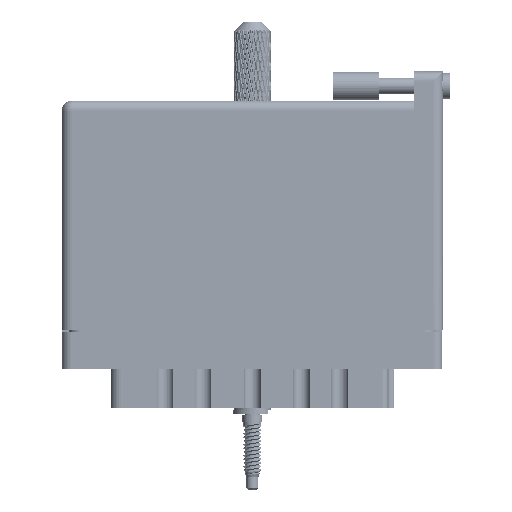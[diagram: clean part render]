
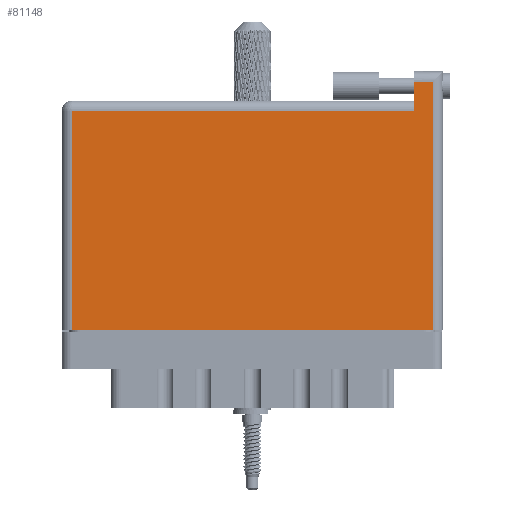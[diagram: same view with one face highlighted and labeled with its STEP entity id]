
A CAD part, front view. The second image highlights one B-rep face of the part: STEP entity #81148.
In plain terms, the highlighted face is planar.
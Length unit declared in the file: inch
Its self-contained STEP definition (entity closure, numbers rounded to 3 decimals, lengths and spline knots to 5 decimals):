
#1826 = AXIS2_PLACEMENT_3D ( 'NONE', #82770, #83542, #58306 ) ;
#6458 = ORIENTED_EDGE ( 'NONE', *, *, #20138, .T. ) ;
#6482 = CARTESIAN_POINT ( 'NONE',  ( 2.53, 1.696, 0. ) ) ;
#8114 = VERTEX_POINT ( 'NONE', #28756 ) ;
#8394 = VERTEX_POINT ( 'NONE', #106217 ) ;
#8810 = EDGE_LOOP ( 'NONE', ( #108241, #108250, #6458, #107707, #86472, #81089 ) ) ;
#10524 = VERTEX_POINT ( 'NONE', #55354 ) ;
#12526 = DIRECTION ( 'NONE',  ( 0., 1., 0. ) ) ;
#14094 = CARTESIAN_POINT ( 'NONE',  ( 0.07, 0., 0. ) ) ;
#14595 = LINE ( 'NONE', #22500, #80674 ) ;
#17447 = DIRECTION ( 'NONE',  ( 0., -1., 0. ) ) ;
#20138 = EDGE_CURVE ( 'NONE', #86736, #8394, #29441, .T. ) ;
#22500 = CARTESIAN_POINT ( 'NONE',  ( 2.53, 1.766, 0. ) ) ;
#27860 = LINE ( 'NONE', #66190, #40802 ) ;
#28756 = CARTESIAN_POINT ( 'NONE',  ( 2.53, 0., 0. ) ) ;
#29441 = LINE ( 'NONE', #54381, #75529 ) ;
#33215 = VERTEX_POINT ( 'NONE', #49548 ) ;
#36217 = LINE ( 'NONE', #70089, #112387 ) ;
#38196 = LINE ( 'NONE', #14094, #77032 ) ;
#40200 = DIRECTION ( 'NONE',  ( 0., -1., 0. ) ) ;
#40802 = VECTOR ( 'NONE', #86658, 39.37008 ) ;
#43495 = EDGE_CURVE ( 'NONE', #10524, #49974, #38196, .T. ) ;
#49107 = PLANE ( 'NONE',  #1826 ) ;
#49548 = CARTESIAN_POINT ( 'NONE',  ( 2.403, 1.496, 0. ) ) ;
#49974 = VERTEX_POINT ( 'NONE', #74102 ) ;
#53403 = VECTOR ( 'NONE', #75954, 39.37008 ) ;
#54381 = CARTESIAN_POINT ( 'NONE',  ( 0., 1.696, 0. ) ) ;
#54705 = FACE_OUTER_BOUND ( 'NONE', #8810, .T. ) ;
#55354 = CARTESIAN_POINT ( 'NONE',  ( 0.07, 1.496, 0. ) ) ;
#57120 = CARTESIAN_POINT ( 'NONE',  ( 0., 1.496, 0. ) ) ;
#58306 = DIRECTION ( 'NONE',  ( -1., 0., 0. ) ) ;
#60147 = EDGE_CURVE ( 'NONE', #49974, #8114, #27860, .T. ) ;
#65885 = EDGE_CURVE ( 'NONE', #8394, #33215, #36217, .T. ) ;
#66190 = CARTESIAN_POINT ( 'NONE',  ( 0., 0., 0. ) ) ;
#67354 = EDGE_CURVE ( 'NONE', #33215, #10524, #74939, .T. ) ;
#70089 = CARTESIAN_POINT ( 'NONE',  ( 2.403, 1.766, 0. ) ) ;
#74102 = CARTESIAN_POINT ( 'NONE',  ( 0.07, 0., 0. ) ) ;
#74939 = LINE ( 'NONE', #57120, #53403 ) ;
#75529 = VECTOR ( 'NONE', #118682, 39.37008 ) ;
#75954 = DIRECTION ( 'NONE',  ( -1., 0., 0. ) ) ;
#77032 = VECTOR ( 'NONE', #40200, 39.37008 ) ;
#78904 = EDGE_CURVE ( 'NONE', #8114, #86736, #14595, .T. ) ;
#80674 = VECTOR ( 'NONE', #12526, 39.37008 ) ;
#81089 = ORIENTED_EDGE ( 'NONE', *, *, #43495, .T. ) ;
#81148 = ADVANCED_FACE ( 'NONE', ( #54705 ), #49107, .F. ) ;
#82770 = CARTESIAN_POINT ( 'NONE',  ( 0., 1.566, 0. ) ) ;
#83542 = DIRECTION ( 'NONE',  ( 0., 0., -1. ) ) ;
#86472 = ORIENTED_EDGE ( 'NONE', *, *, #67354, .T. ) ;
#86658 = DIRECTION ( 'NONE',  ( 1., 0., 0. ) ) ;
#86736 = VERTEX_POINT ( 'NONE', #6482 ) ;
#106217 = CARTESIAN_POINT ( 'NONE',  ( 2.403, 1.696, 0. ) ) ;
#107707 = ORIENTED_EDGE ( 'NONE', *, *, #65885, .T. ) ;
#108241 = ORIENTED_EDGE ( 'NONE', *, *, #60147, .T. ) ;
#108250 = ORIENTED_EDGE ( 'NONE', *, *, #78904, .T. ) ;
#112387 = VECTOR ( 'NONE', #17447, 39.37008 ) ;
#118682 = DIRECTION ( 'NONE',  ( -1., 0., 0. ) ) ;
